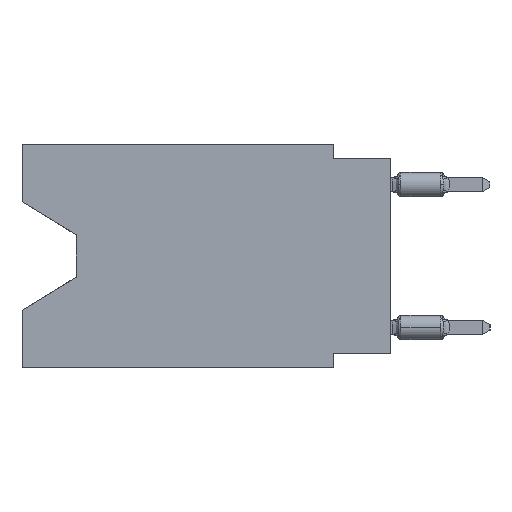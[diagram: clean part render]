
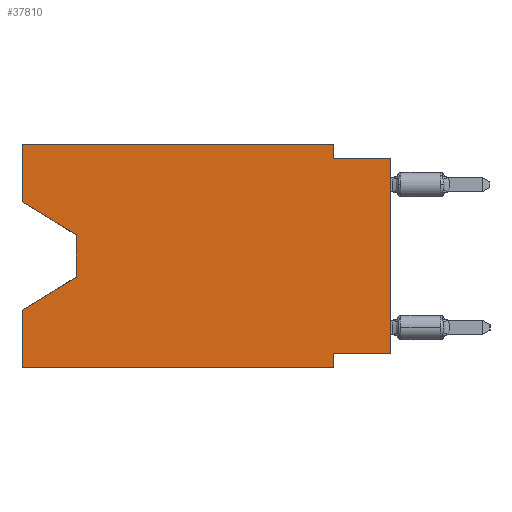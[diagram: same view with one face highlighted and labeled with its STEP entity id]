
A CAD part, left-side view. The second image highlights one B-rep face of the part: STEP entity #37810.
In plain terms, the highlighted planar face has unit normal (-1, 0, 0).
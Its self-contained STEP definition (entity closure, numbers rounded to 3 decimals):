
#2 = LINE ( 'NONE', #40557, #12067 ) ;
#45 = EDGE_CURVE ( 'NONE', #37408, #39245, #35623, .T. ) ;
#108 = LINE ( 'NONE', #16510, #7887 ) ;
#473 = CARTESIAN_POINT ( 'NONE',  ( 0., 16.383, 0. ) ) ;
#2284 = CARTESIAN_POINT ( 'NONE',  ( 0., 16.383, 0. ) ) ;
#3621 = DIRECTION ( 'NONE',  ( 0., -0.855, -0.519 ) ) ;
#3834 = CARTESIAN_POINT ( 'NONE',  ( 0., 13.97, -4.013 ) ) ;
#4501 = EDGE_LOOP ( 'NONE', ( #35221, #31153, #15571, #42741, #9513, #34140, #5305, #24846, #20608, #9316, #8094, #35079 ) ) ;
#4907 = VERTEX_POINT ( 'NONE', #2284 ) ;
#5254 = DIRECTION ( 'NONE',  ( 0., 0.855, -0.519 ) ) ;
#5305 = ORIENTED_EDGE ( 'NONE', *, *, #30309, .F. ) ;
#5408 = LINE ( 'NONE', #39964, #7350 ) ;
#5875 = VECTOR ( 'NONE', #6221, 1000. ) ;
#6120 = EDGE_CURVE ( 'NONE', #30060, #16473, #18924, .T. ) ;
#6221 = DIRECTION ( 'NONE',  ( 0., 0., -1. ) ) ;
#6756 = EDGE_CURVE ( 'NONE', #4907, #42690, #23944, .T. ) ;
#6903 = DIRECTION ( 'NONE',  ( 0., -1., 0. ) ) ;
#7350 = VECTOR ( 'NONE', #29565, 1000. ) ;
#7418 = EDGE_CURVE ( 'NONE', #26480, #16473, #5408, .T. ) ;
#7887 = VECTOR ( 'NONE', #30463, 1000. ) ;
#8094 = ORIENTED_EDGE ( 'NONE', *, *, #6756, .F. ) ;
#9109 = EDGE_CURVE ( 'NONE', #20424, #39245, #15523, .T. ) ;
#9316 = ORIENTED_EDGE ( 'NONE', *, *, #27484, .F. ) ;
#9513 = ORIENTED_EDGE ( 'NONE', *, *, #19026, .T. ) ;
#9536 = VECTOR ( 'NONE', #17350, 1000. ) ;
#10138 = EDGE_CURVE ( 'NONE', #16679, #35481, #41285, .T. ) ;
#10928 = CARTESIAN_POINT ( 'NONE',  ( 0., 16.383, -2.546 ) ) ;
#10971 = VECTOR ( 'NONE', #5254, 1000. ) ;
#11098 = LINE ( 'NONE', #14838, #42512 ) ;
#12067 = VECTOR ( 'NONE', #15030, 1000. ) ;
#12883 = FACE_OUTER_BOUND ( 'NONE', #4501, .T. ) ;
#13783 = CARTESIAN_POINT ( 'NONE',  ( 0., 2.54, -9.271 ) ) ;
#14210 = LINE ( 'NONE', #3834, #9536 ) ;
#14835 = CARTESIAN_POINT ( 'NONE',  ( 0., 16.383, -2.546 ) ) ;
#14838 = CARTESIAN_POINT ( 'NONE',  ( 0., 16.383, -9.906 ) ) ;
#15030 = DIRECTION ( 'NONE',  ( 0., 1., 0. ) ) ;
#15523 = LINE ( 'NONE', #29063, #17254 ) ;
#15571 = ORIENTED_EDGE ( 'NONE', *, *, #45, .T. ) ;
#16167 = CARTESIAN_POINT ( 'NONE',  ( 0., 2.54, -9.906 ) ) ;
#16313 = CARTESIAN_POINT ( 'NONE',  ( 0., 2.54, 0. ) ) ;
#16473 = VERTEX_POINT ( 'NONE', #36623 ) ;
#16510 = CARTESIAN_POINT ( 'NONE',  ( 0., 16.383, 0. ) ) ;
#16679 = VERTEX_POINT ( 'NONE', #14835 ) ;
#17254 = VECTOR ( 'NONE', #39246, 1000. ) ;
#17350 = DIRECTION ( 'NONE',  ( 0., 0., -1. ) ) ;
#18150 = DIRECTION ( 'NONE',  ( 0., 0., -1. ) ) ;
#18924 = LINE ( 'NONE', #35791, #35683 ) ;
#19026 = EDGE_CURVE ( 'NONE', #20424, #30882, #11098, .T. ) ;
#20424 = VERTEX_POINT ( 'NONE', #31976 ) ;
#20608 = ORIENTED_EDGE ( 'NONE', *, *, #7418, .F. ) ;
#21988 = VERTEX_POINT ( 'NONE', #13783 ) ;
#22260 = EDGE_CURVE ( 'NONE', #21988, #30882, #23058, .T. ) ;
#23058 = LINE ( 'NONE', #16167, #5875 ) ;
#23944 = LINE ( 'NONE', #473, #37030 ) ;
#24846 = ORIENTED_EDGE ( 'NONE', *, *, #6120, .T. ) ;
#25213 = CARTESIAN_POINT ( 'NONE',  ( 0., 13.97, -5.893 ) ) ;
#26433 = DIRECTION ( 'NONE',  ( 1., 0., 0. ) ) ;
#26480 = VERTEX_POINT ( 'NONE', #31664 ) ;
#27328 = PLANE ( 'NONE',  #37606 ) ;
#27484 = EDGE_CURVE ( 'NONE', #42690, #26480, #31672, .T. ) ;
#29063 = CARTESIAN_POINT ( 'NONE',  ( 0., 16.383, 0. ) ) ;
#29565 = DIRECTION ( 'NONE',  ( 0., -1., 0. ) ) ;
#30060 = VERTEX_POINT ( 'NONE', #31724 ) ;
#30309 = EDGE_CURVE ( 'NONE', #30060, #21988, #2, .T. ) ;
#30448 = CARTESIAN_POINT ( 'NONE',  ( 0., 13.97, -5.893 ) ) ;
#30463 = DIRECTION ( 'NONE',  ( 0., 0., 1. ) ) ;
#30882 = VERTEX_POINT ( 'NONE', #42674 ) ;
#30981 = EDGE_CURVE ( 'NONE', #16679, #4907, #108, .T. ) ;
#31153 = ORIENTED_EDGE ( 'NONE', *, *, #41521, .T. ) ;
#31265 = CARTESIAN_POINT ( 'NONE',  ( 0., 16.383, -7.36 ) ) ;
#31664 = CARTESIAN_POINT ( 'NONE',  ( 0., 2.54, -0.635 ) ) ;
#31672 = LINE ( 'NONE', #38524, #41246 ) ;
#31724 = CARTESIAN_POINT ( 'NONE',  ( 0., 0., -9.271 ) ) ;
#31976 = CARTESIAN_POINT ( 'NONE',  ( 0., 16.383, -9.906 ) ) ;
#34140 = ORIENTED_EDGE ( 'NONE', *, *, #22260, .F. ) ;
#34736 = CARTESIAN_POINT ( 'NONE',  ( 0., 13.97, -4.013 ) ) ;
#35079 = ORIENTED_EDGE ( 'NONE', *, *, #30981, .F. ) ;
#35221 = ORIENTED_EDGE ( 'NONE', *, *, #10138, .T. ) ;
#35481 = VERTEX_POINT ( 'NONE', #34736 ) ;
#35623 = LINE ( 'NONE', #25213, #10971 ) ;
#35683 = VECTOR ( 'NONE', #42633, 1000. ) ;
#35791 = CARTESIAN_POINT ( 'NONE',  ( 0., 0., 0. ) ) ;
#36623 = CARTESIAN_POINT ( 'NONE',  ( 0., 0., -0.635 ) ) ;
#36633 = DIRECTION ( 'NONE',  ( 0., 0., -1. ) ) ;
#37030 = VECTOR ( 'NONE', #6903, 1000. ) ;
#37408 = VERTEX_POINT ( 'NONE', #30448 ) ;
#37606 = AXIS2_PLACEMENT_3D ( 'NONE', #43725, #26433, #36633 ) ;
#37810 = ADVANCED_FACE ( 'NONE', ( #12883 ), #27328, .F. ) ;
#38524 = CARTESIAN_POINT ( 'NONE',  ( 0., 2.54, 0. ) ) ;
#38527 = VECTOR ( 'NONE', #3621, 1000. ) ;
#39245 = VERTEX_POINT ( 'NONE', #31265 ) ;
#39246 = DIRECTION ( 'NONE',  ( 0., 0., 1. ) ) ;
#39964 = CARTESIAN_POINT ( 'NONE',  ( 0., 0., -0.635 ) ) ;
#40557 = CARTESIAN_POINT ( 'NONE',  ( 0., 0., -9.271 ) ) ;
#41235 = DIRECTION ( 'NONE',  ( 0., -1., 0. ) ) ;
#41246 = VECTOR ( 'NONE', #18150, 1000. ) ;
#41285 = LINE ( 'NONE', #10928, #38527 ) ;
#41521 = EDGE_CURVE ( 'NONE', #35481, #37408, #14210, .T. ) ;
#42512 = VECTOR ( 'NONE', #41235, 1000. ) ;
#42633 = DIRECTION ( 'NONE',  ( 0., 0., 1. ) ) ;
#42674 = CARTESIAN_POINT ( 'NONE',  ( 0., 2.54, -9.906 ) ) ;
#42690 = VERTEX_POINT ( 'NONE', #16313 ) ;
#42741 = ORIENTED_EDGE ( 'NONE', *, *, #9109, .F. ) ;
#43725 = CARTESIAN_POINT ( 'NONE',  ( 0., 16.383, 0. ) ) ;
